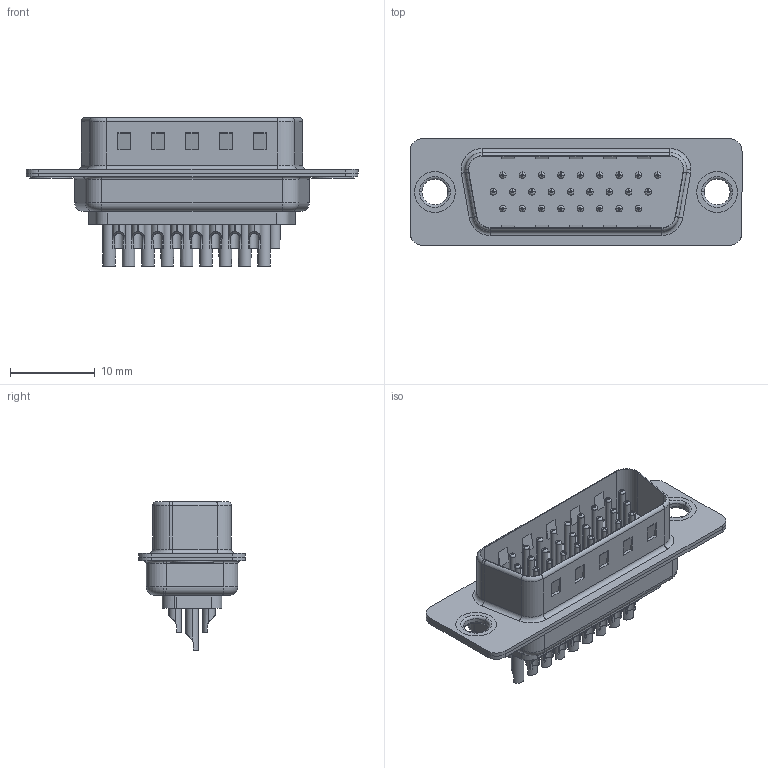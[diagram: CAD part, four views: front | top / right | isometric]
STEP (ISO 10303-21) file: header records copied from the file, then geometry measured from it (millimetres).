
FILE_DESCRIPTION (( 'STEP AP203' ), '1' );
FILE_NAME ('637-026-332-261.STEP', '2020-07-18T01:05:40', ( '' ), ( '' ), 'SwSTEP 2.0', 'SolidWorks 2020', '' );
FILE_SCHEMA (( 'CONFIG_CONTROL_DESIGN' ));
Length unit declared in the file: millimetre
Products named in the file (8): 637 Contact Row 2_32; 637 Shell Rear_26 Contacts; 637 Housing_26 Contacts; 637-026-332-261; 637 Shell Front_26 Contacts; 637 Thru Hole Rivet; 637 Contact Row 1_32; 637 Contact Row 3_32
Assembly tree (31 placements, depth 2):
  637-026-332-261
    637 Housing_26 Contacts
    637 Shell Front_26 Contacts
    637 Shell Rear_26 Contacts
    637 Contact Row 1_32  x9
    637 Contact Row 2_32  x9
    637 Contact Row 3_32  x8
    637 Thru Hole Rivet  x2
Bounding box: 39.2 x 12.6 x 17.55 mm (x, y, z)
Volume: 1776.5 mm3; surface area: 6780.9 mm2
Topology: 31 solids, 31 shells, 1978 faces, 5039 edges, 3186 vertices
Faces by surface type: cylinder 871, torus 604, plane 503
Entity records: 21808 total; most frequent: DIRECTION 3847, CARTESIAN_POINT 3581, ORIENTED_EDGE 3282, EDGE_CURVE 1641, AXIS2_PLACEMENT_3D 1553, VERTEX_POINT 1046, CIRCLE 849, EDGE_LOOP 817
